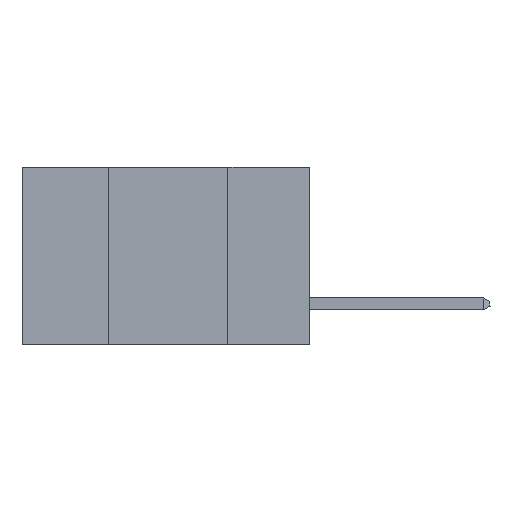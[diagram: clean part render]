
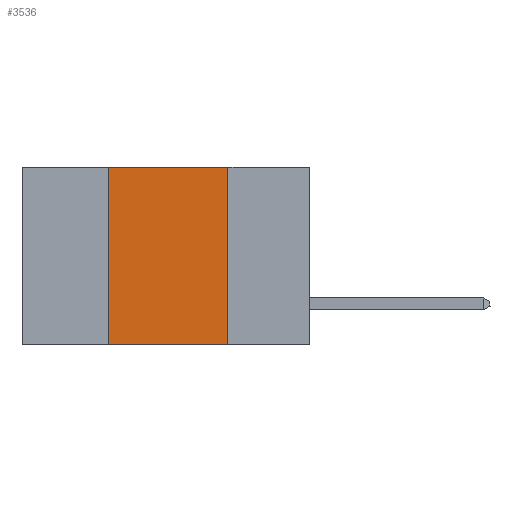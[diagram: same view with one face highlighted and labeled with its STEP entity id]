
A CAD part, left-side view. The second image highlights one B-rep face of the part: STEP entity #3536.
In plain terms, the highlighted planar face has unit normal (-1, 0, 0).
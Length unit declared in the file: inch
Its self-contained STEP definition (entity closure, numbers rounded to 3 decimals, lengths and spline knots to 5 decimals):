
#1410 = VECTOR ( 'NONE', #15588, 39.37008 ) ;
#1732 = VERTEX_POINT ( 'NONE', #2173 ) ;
#1755 = CARTESIAN_POINT ( 'NONE',  ( 0., 0.17, 0. ) ) ;
#1994 = ORIENTED_EDGE ( 'NONE', *, *, #24490, .F. ) ;
#2173 = CARTESIAN_POINT ( 'NONE',  ( 0., 0.42, -0.37 ) ) ;
#2595 = DIRECTION ( 'NONE',  ( 0., -1., 0. ) ) ;
#3499 = DIRECTION ( 'NONE',  ( 0., -1., 0. ) ) ;
#3536 = ADVANCED_FACE ( 'NONE', ( #10134 ), #21000, .F. ) ;
#3583 = ORIENTED_EDGE ( 'NONE', *, *, #8553, .F. ) ;
#4307 = VERTEX_POINT ( 'NONE', #1755 ) ;
#5382 = CARTESIAN_POINT ( 'NONE',  ( 0., 0.42, 0. ) ) ;
#5826 = ORIENTED_EDGE ( 'NONE', *, *, #27913, .F. ) ;
#7518 = DIRECTION ( 'NONE',  ( 0., 0., 1. ) ) ;
#7870 = LINE ( 'NONE', #25341, #1410 ) ;
#7949 = VERTEX_POINT ( 'NONE', #24064 ) ;
#8334 = CARTESIAN_POINT ( 'NONE',  ( 0., 0.6, 0. ) ) ;
#8553 = EDGE_CURVE ( 'NONE', #4307, #7949, #7870, .T. ) ;
#8893 = VECTOR ( 'NONE', #3499, 39.37008 ) ;
#10134 = FACE_OUTER_BOUND ( 'NONE', #13655, .T. ) ;
#10817 = DIRECTION ( 'NONE',  ( 1., 0., 0. ) ) ;
#10861 = ORIENTED_EDGE ( 'NONE', *, *, #28565, .T. ) ;
#11996 = CARTESIAN_POINT ( 'NONE',  ( 0., 0.6, -0.37 ) ) ;
#13426 = LINE ( 'NONE', #11996, #17635 ) ;
#13483 = LINE ( 'NONE', #22648, #8893 ) ;
#13655 = EDGE_LOOP ( 'NONE', ( #3583, #1994, #5826, #10861 ) ) ;
#13856 = LINE ( 'NONE', #24887, #19624 ) ;
#15588 = DIRECTION ( 'NONE',  ( 0., 0., -1. ) ) ;
#15726 = DIRECTION ( 'NONE',  ( 0., 0., -1. ) ) ;
#17635 = VECTOR ( 'NONE', #2595, 39.37008 ) ;
#19624 = VECTOR ( 'NONE', #7518, 39.37008 ) ;
#21000 = PLANE ( 'NONE',  #29799 ) ;
#22648 = CARTESIAN_POINT ( 'NONE',  ( 0., 0.6, 0. ) ) ;
#24064 = CARTESIAN_POINT ( 'NONE',  ( 0., 0.17, -0.37 ) ) ;
#24490 = EDGE_CURVE ( 'NONE', #24579, #4307, #13483, .T. ) ;
#24579 = VERTEX_POINT ( 'NONE', #5382 ) ;
#24887 = CARTESIAN_POINT ( 'NONE',  ( 0., 0.42, 0. ) ) ;
#25341 = CARTESIAN_POINT ( 'NONE',  ( 0., 0.17, 0. ) ) ;
#27913 = EDGE_CURVE ( 'NONE', #1732, #24579, #13856, .T. ) ;
#28565 = EDGE_CURVE ( 'NONE', #1732, #7949, #13426, .T. ) ;
#29799 = AXIS2_PLACEMENT_3D ( 'NONE', #8334, #10817, #15726 ) ;
